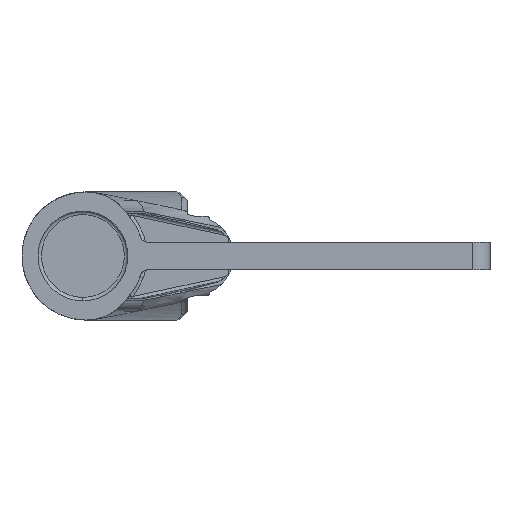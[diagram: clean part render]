
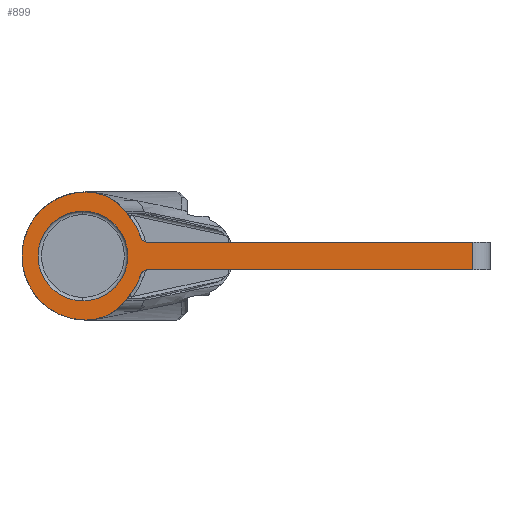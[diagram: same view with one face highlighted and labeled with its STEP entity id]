
A CAD part, left-side view. The second image highlights one B-rep face of the part: STEP entity #899.
In plain terms, the highlighted planar face has unit normal (-1, 0, 0).
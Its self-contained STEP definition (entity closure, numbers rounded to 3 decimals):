
#48 = DIRECTION ( 'NONE',  ( 0., 0., -1. ) ) ;
#49 = EDGE_LOOP ( 'NONE', ( #6295, #6751, #5604, #2349, #5627, #5974, #3216, #2139, #1667, #1520, #3123 ) ) ;
#71 = AXIS2_PLACEMENT_3D ( 'NONE', #2912, #1843, #2376 ) ;
#151 = CARTESIAN_POINT ( 'NONE',  ( -422.78, 21.427, 18.567 ) ) ;
#231 = CARTESIAN_POINT ( 'NONE',  ( -422.78, 36.178, -11.521 ) ) ;
#302 = CARTESIAN_POINT ( 'NONE',  ( -422.78, 39.991, 1.368 ) ) ;
#489 = AXIS2_PLACEMENT_3D ( 'NONE', #5043, #877, #5609 ) ;
#510 = DIRECTION ( 'NONE',  ( 0., 0., 1. ) ) ;
#577 = FACE_OUTER_BOUND ( 'NONE', #49, .T. ) ;
#667 = LINE ( 'NONE', #3989, #2433 ) ;
#675 = DIRECTION ( 'NONE',  ( -1., 0., 0. ) ) ;
#689 = CARTESIAN_POINT ( 'NONE',  ( -422.78, 39.991, -1.368 ) ) ;
#759 = CARTESIAN_POINT ( 'NONE',  ( -422.78, 39.991, 0. ) ) ;
#771 = EDGE_CURVE ( 'NONE', #5495, #2787, #1831, .T. ) ;
#823 = CARTESIAN_POINT ( 'NONE',  ( -422.78, 33.294, 14.475 ) ) ;
#830 = VERTEX_POINT ( 'NONE', #4321 ) ;
#877 = DIRECTION ( 'NONE',  ( -1., 0., 0. ) ) ;
#899 = ADVANCED_FACE ( 'NONE', ( #577, #6936 ), #2102, .F. ) ;
#908 = EDGE_CURVE ( 'NONE', #6367, #3885, #2086, .T. ) ;
#1047 = EDGE_CURVE ( 'NONE', #3442, #3287, #4448, .T. ) ;
#1138 = DIRECTION ( 'NONE',  ( 0., 0., 1. ) ) ;
#1144 = CIRCLE ( 'NONE', #1946, 13. ) ;
#1251 = DIRECTION ( 'NONE',  ( 0., 0., -1. ) ) ;
#1254 = CARTESIAN_POINT ( 'NONE',  ( -422.78, 21.574, -18.567 ) ) ;
#1285 = ORIENTED_EDGE ( 'NONE', *, *, #3118, .F. ) ;
#1366 = DIRECTION ( 'NONE',  ( 0., 0., 1. ) ) ;
#1391 = CARTESIAN_POINT ( 'NONE',  ( -422.78, 21.574, 18.567 ) ) ;
#1402 = AXIS2_PLACEMENT_3D ( 'NONE', #6638, #675, #2834 ) ;
#1465 = CARTESIAN_POINT ( 'NONE',  ( -422.78, 21.427, 18.567 ) ) ;
#1520 = ORIENTED_EDGE ( 'NONE', *, *, #6405, .T. ) ;
#1573 = DIRECTION ( 'NONE',  ( 1., 0., 0. ) ) ;
#1667 = ORIENTED_EDGE ( 'NONE', *, *, #771, .T. ) ;
#1831 = B_SPLINE_CURVE_WITH_KNOTS ( 'NONE', 3,
 ( #1465, #1391, #4045, #6197, #5666, #823, #2990, #5135, #5171, #302, #1959 ),
 .UNSPECIFIED., .F., .F.,
 ( 4, 1, 1, 1, 1, 1, 1, 1, 4 ),
 ( 0.056, 0.057, 0.061, 0.064, 0.068, 0.072, 0.076, 0.08, 0.084 ),
 .UNSPECIFIED. ) ;
#1843 = DIRECTION ( 'NONE',  ( -1., 0., 0. ) ) ;
#1871 = AXIS2_PLACEMENT_3D ( 'NONE', #2172, #3871, #1138 ) ;
#1880 = AXIS2_PLACEMENT_3D ( 'NONE', #3425, #4639, #1251 ) ;
#1946 = AXIS2_PLACEMENT_3D ( 'NONE', #2437, #6772, #1366 ) ;
#1959 = CARTESIAN_POINT ( 'NONE',  ( -422.78, 39.991, 0. ) ) ;
#2061 = CIRCLE ( 'NONE', #489, 17.641 ) ;
#2086 = CIRCLE ( 'NONE', #6023, 2. ) ;
#2102 = PLANE ( 'NONE',  #6817 ) ;
#2139 = ORIENTED_EDGE ( 'NONE', *, *, #4292, .F. ) ;
#2166 = EDGE_CURVE ( 'NONE', #830, #6080, #667, .T. ) ;
#2172 = CARTESIAN_POINT ( 'NONE',  ( -422.78, 21.427, -4.109 ) ) ;
#2226 = AXIS2_PLACEMENT_3D ( 'NONE', #4110, #5349, #510 ) ;
#2349 = ORIENTED_EDGE ( 'NONE', *, *, #4397, .F. ) ;
#2376 = DIRECTION ( 'NONE',  ( 0., 0., 1. ) ) ;
#2427 = CARTESIAN_POINT ( 'NONE',  ( -422.78, 33.294, -14.475 ) ) ;
#2433 = VECTOR ( 'NONE', #3372, 1000. ) ;
#2437 = CARTESIAN_POINT ( 'NONE',  ( -422.78, 22.35, 0. ) ) ;
#2444 = CIRCLE ( 'NONE', #71, 13. ) ;
#2492 = DIRECTION ( 'NONE',  ( 0., 0., -1. ) ) ;
#2526 = CARTESIAN_POINT ( 'NONE',  ( -422.78, 39.991, 0. ) ) ;
#2627 = CARTESIAN_POINT ( 'NONE',  ( -422.78, 5.552, -5.389 ) ) ;
#2787 = VERTEX_POINT ( 'NONE', #2526 ) ;
#2802 = B_SPLINE_CURVE_WITH_KNOTS ( 'NONE', 3,
 ( #759, #689, #3980, #2922, #231, #2427, #2958, #6165, #5106, #1254, #2850 ),
 .UNSPECIFIED., .F., .F.,
 ( 4, 1, 1, 1, 1, 1, 1, 1, 4 ),
 ( 0., 0.004, 0.008, 0.012, 0.016, 0.02, 0.025, 0.029, 0.029 ),
 .UNSPECIFIED. ) ;
#2834 = DIRECTION ( 'NONE',  ( 0., 0., 1. ) ) ;
#2850 = CARTESIAN_POINT ( 'NONE',  ( -422.78, 21.427, -18.567 ) ) ;
#2851 = EDGE_CURVE ( 'NONE', #3442, #6087, #3244, .T. ) ;
#2899 = VERTEX_POINT ( 'NONE', #3350 ) ;
#2912 = CARTESIAN_POINT ( 'NONE',  ( -422.78, 22.35, 0. ) ) ;
#2922 = CARTESIAN_POINT ( 'NONE',  ( -422.78, 38.344, -8.007 ) ) ;
#2958 = CARTESIAN_POINT ( 'NONE',  ( -422.78, 29.832, -16.724 ) ) ;
#2990 = CARTESIAN_POINT ( 'NONE',  ( -422.78, 36.178, 11.521 ) ) ;
#3007 = CARTESIAN_POINT ( 'NONE',  ( -422.78, 21.427, -18.567 ) ) ;
#3118 = EDGE_CURVE ( 'NONE', #2899, #3851, #2444, .T. ) ;
#3123 = ORIENTED_EDGE ( 'NONE', *, *, #2851, .F. ) ;
#3167 = CARTESIAN_POINT ( 'NONE',  ( -422.78, 39.991, -23.02 ) ) ;
#3206 = DIRECTION ( 'NONE',  ( 0., 0., -1. ) ) ;
#3216 = ORIENTED_EDGE ( 'NONE', *, *, #6948, .T. ) ;
#3244 = CIRCLE ( 'NONE', #1871, 14.458 ) ;
#3287 = VERTEX_POINT ( 'NONE', #2627 ) ;
#3350 = CARTESIAN_POINT ( 'NONE',  ( -422.78, 22.35, -13. ) ) ;
#3372 = DIRECTION ( 'NONE',  ( 0., -1., 0. ) ) ;
#3425 = CARTESIAN_POINT ( 'NONE',  ( -422.78, 3.647, -6. ) ) ;
#3442 = VERTEX_POINT ( 'NONE', #3962 ) ;
#3709 = VECTOR ( 'NONE', #2492, 1000. ) ;
#3725 = ORIENTED_EDGE ( 'NONE', *, *, #6170, .F. ) ;
#3816 = CIRCLE ( 'NONE', #1880, 2. ) ;
#3851 = VERTEX_POINT ( 'NONE', #6661 ) ;
#3871 = DIRECTION ( 'NONE',  ( 1., 0., 0. ) ) ;
#3885 = VERTEX_POINT ( 'NONE', #5716 ) ;
#3923 = CARTESIAN_POINT ( 'NONE',  ( -422.78, -90.65, -4. ) ) ;
#3962 = CARTESIAN_POINT ( 'NONE',  ( -422.78, 9.069, -11.612 ) ) ;
#3980 = CARTESIAN_POINT ( 'NONE',  ( -422.78, 39.688, -4.103 ) ) ;
#3989 = CARTESIAN_POINT ( 'NONE',  ( -422.78, 9.35, -4. ) ) ;
#4004 = CARTESIAN_POINT ( 'NONE',  ( -422.78, -90.65, 4. ) ) ;
#4045 = CARTESIAN_POINT ( 'NONE',  ( -422.78, 23.088, 18.549 ) ) ;
#4110 = CARTESIAN_POINT ( 'NONE',  ( -422.78, 21.427, 4.109 ) ) ;
#4292 = EDGE_CURVE ( 'NONE', #5495, #4314, #6283, .T. ) ;
#4314 = VERTEX_POINT ( 'NONE', #6972 ) ;
#4321 = CARTESIAN_POINT ( 'NONE',  ( -422.78, 3.647, -4. ) ) ;
#4326 = EDGE_CURVE ( 'NONE', #3287, #830, #3816, .T. ) ;
#4397 = EDGE_CURVE ( 'NONE', #6610, #6080, #5030, .T. ) ;
#4427 = LINE ( 'NONE', #6643, #5088 ) ;
#4448 = CIRCLE ( 'NONE', #1402, 17.641 ) ;
#4639 = DIRECTION ( 'NONE',  ( 1., 0., 0. ) ) ;
#5006 = EDGE_LOOP ( 'NONE', ( #3725, #1285 ) ) ;
#5030 = LINE ( 'NONE', #5668, #3709 ) ;
#5043 = CARTESIAN_POINT ( 'NONE',  ( -422.78, 22.35, 0. ) ) ;
#5088 = VECTOR ( 'NONE', #6576, 1000. ) ;
#5106 = CARTESIAN_POINT ( 'NONE',  ( -422.78, 23.088, -18.549 ) ) ;
#5135 = CARTESIAN_POINT ( 'NONE',  ( -422.78, 38.344, 8.007 ) ) ;
#5171 = CARTESIAN_POINT ( 'NONE',  ( -422.78, 39.688, 4.103 ) ) ;
#5349 = DIRECTION ( 'NONE',  ( 1., 0., 0. ) ) ;
#5388 = DIRECTION ( 'NONE',  ( 1., 0., 0. ) ) ;
#5495 = VERTEX_POINT ( 'NONE', #151 ) ;
#5526 = EDGE_CURVE ( 'NONE', #6367, #6610, #4427, .T. ) ;
#5532 = CARTESIAN_POINT ( 'NONE',  ( -422.78, 3.647, 4. ) ) ;
#5604 = ORIENTED_EDGE ( 'NONE', *, *, #2166, .T. ) ;
#5609 = DIRECTION ( 'NONE',  ( 0., 0., 1. ) ) ;
#5627 = ORIENTED_EDGE ( 'NONE', *, *, #5526, .F. ) ;
#5666 = CARTESIAN_POINT ( 'NONE',  ( -422.78, 29.832, 16.724 ) ) ;
#5668 = CARTESIAN_POINT ( 'NONE',  ( -422.78, -90.65, 4. ) ) ;
#5716 = CARTESIAN_POINT ( 'NONE',  ( -422.78, 5.552, 5.389 ) ) ;
#5912 = CARTESIAN_POINT ( 'NONE',  ( -422.78, 3.647, 6. ) ) ;
#5974 = ORIENTED_EDGE ( 'NONE', *, *, #908, .T. ) ;
#6023 = AXIS2_PLACEMENT_3D ( 'NONE', #5912, #5388, #48 ) ;
#6080 = VERTEX_POINT ( 'NONE', #3923 ) ;
#6087 = VERTEX_POINT ( 'NONE', #3007 ) ;
#6165 = CARTESIAN_POINT ( 'NONE',  ( -422.78, 25.962, -18.16 ) ) ;
#6170 = EDGE_CURVE ( 'NONE', #3851, #2899, #1144, .T. ) ;
#6197 = CARTESIAN_POINT ( 'NONE',  ( -422.78, 25.962, 18.16 ) ) ;
#6283 = CIRCLE ( 'NONE', #2226, 14.458 ) ;
#6295 = ORIENTED_EDGE ( 'NONE', *, *, #1047, .T. ) ;
#6367 = VERTEX_POINT ( 'NONE', #5532 ) ;
#6405 = EDGE_CURVE ( 'NONE', #2787, #6087, #2802, .T. ) ;
#6576 = DIRECTION ( 'NONE',  ( 0., -1., 0. ) ) ;
#6610 = VERTEX_POINT ( 'NONE', #4004 ) ;
#6638 = CARTESIAN_POINT ( 'NONE',  ( -422.78, 22.35, 0. ) ) ;
#6643 = CARTESIAN_POINT ( 'NONE',  ( -422.78, 9.35, 4. ) ) ;
#6661 = CARTESIAN_POINT ( 'NONE',  ( -422.78, 22.35, 13. ) ) ;
#6751 = ORIENTED_EDGE ( 'NONE', *, *, #4326, .T. ) ;
#6772 = DIRECTION ( 'NONE',  ( -1., 0., 0. ) ) ;
#6817 = AXIS2_PLACEMENT_3D ( 'NONE', #3167, #1573, #3206 ) ;
#6936 = FACE_BOUND ( 'NONE', #5006, .T. ) ;
#6948 = EDGE_CURVE ( 'NONE', #3885, #4314, #2061, .T. ) ;
#6972 = CARTESIAN_POINT ( 'NONE',  ( -422.78, 9.069, 11.612 ) ) ;
